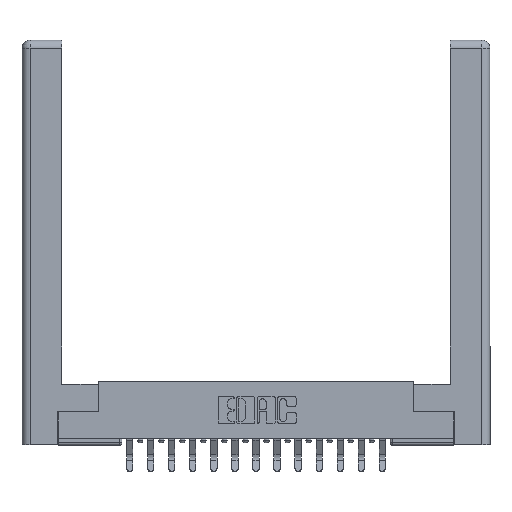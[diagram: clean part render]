
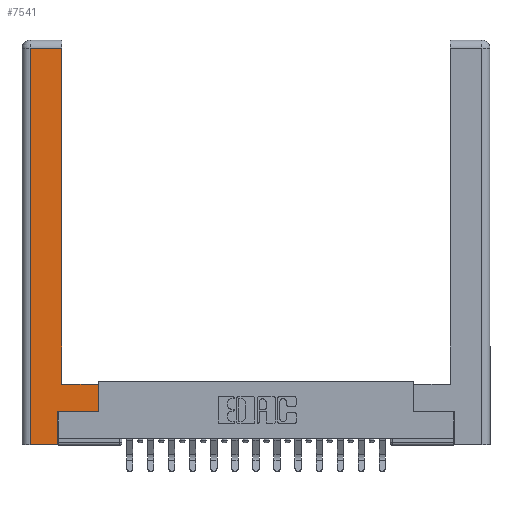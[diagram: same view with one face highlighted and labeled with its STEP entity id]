
A CAD part, top view. The second image highlights one B-rep face of the part: STEP entity #7541.
In plain terms, the highlighted planar face has unit normal (0, 0, 1).
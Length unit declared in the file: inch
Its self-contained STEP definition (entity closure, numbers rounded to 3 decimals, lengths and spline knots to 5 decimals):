
#1090 = AXIS2_PLACEMENT_3D ( 'NONE', #5129, #3698, #3776 ) ;
#1228 = CARTESIAN_POINT ( 'NONE',  ( 0.0615, 2.94, 0. ) ) ;
#1340 = VERTEX_POINT ( 'NONE', #2956 ) ;
#1878 = ORIENTED_EDGE ( 'NONE', *, *, #16406, .T. ) ;
#2419 = PLANE ( 'NONE',  #1090 ) ;
#2557 = VERTEX_POINT ( 'NONE', #12459 ) ;
#2625 = ORIENTED_EDGE ( 'NONE', *, *, #5947, .T. ) ;
#2754 = EDGE_CURVE ( 'NONE', #13485, #1340, #7481, .T. ) ;
#2850 = VECTOR ( 'NONE', #7127, 39.37008 ) ;
#2956 = CARTESIAN_POINT ( 'NONE',  ( 0.265, 0., 0. ) ) ;
#3149 = VERTEX_POINT ( 'NONE', #3576 ) ;
#3239 = ORIENTED_EDGE ( 'NONE', *, *, #15809, .T. ) ;
#3576 = CARTESIAN_POINT ( 'NONE',  ( 0.295, 0.45, 0. ) ) ;
#3641 = DIRECTION ( 'NONE',  ( 0., 1., 0. ) ) ;
#3698 = DIRECTION ( 'NONE',  ( 0., 0., -1. ) ) ;
#3776 = DIRECTION ( 'NONE',  ( -1., 0., 0. ) ) ;
#4039 = ORIENTED_EDGE ( 'NONE', *, *, #4901, .T. ) ;
#4318 = CARTESIAN_POINT ( 'NONE',  ( 0.0615, 0., 0. ) ) ;
#4670 = CARTESIAN_POINT ( 'NONE',  ( 0.565, 0.45, 0. ) ) ;
#4765 = VECTOR ( 'NONE', #6373, 39.37008 ) ;
#4901 = EDGE_CURVE ( 'NONE', #16887, #3149, #8826, .T. ) ;
#4949 = EDGE_LOOP ( 'NONE', ( #3239, #1878, #8077, #7996, #11765, #2625, #17188, #4039 ) ) ;
#5129 = CARTESIAN_POINT ( 'NONE',  ( 0., 0., 0. ) ) ;
#5903 = CARTESIAN_POINT ( 'NONE',  ( 0.0615, 2.94, 0. ) ) ;
#5947 = EDGE_CURVE ( 'NONE', #13837, #2557, #15379, .T. ) ;
#6021 = CARTESIAN_POINT ( 'NONE',  ( 0.295, 0.45, 0. ) ) ;
#6345 = LINE ( 'NONE', #17328, #15395 ) ;
#6373 = DIRECTION ( 'NONE',  ( -1., 0., 0. ) ) ;
#6860 = CARTESIAN_POINT ( 'NONE',  ( 0.565, 0.245, 0. ) ) ;
#7127 = DIRECTION ( 'NONE',  ( 0., -1., 0. ) ) ;
#7481 = LINE ( 'NONE', #15844, #9956 ) ;
#7541 = ADVANCED_FACE ( 'NONE', ( #7837 ), #2419, .F. ) ;
#7837 = FACE_OUTER_BOUND ( 'NONE', #4949, .T. ) ;
#7996 = ORIENTED_EDGE ( 'NONE', *, *, #2754, .T. ) ;
#8077 = ORIENTED_EDGE ( 'NONE', *, *, #8621, .T. ) ;
#8224 = LINE ( 'NONE', #4318, #2850 ) ;
#8266 = VECTOR ( 'NONE', #16744, 39.37008 ) ;
#8571 = DIRECTION ( 'NONE',  ( 0., 1., 0. ) ) ;
#8621 = EDGE_CURVE ( 'NONE', #16716, #13485, #8224, .T. ) ;
#8826 = LINE ( 'NONE', #6021, #4765 ) ;
#8844 = DIRECTION ( 'NONE',  ( 0., 1., 0. ) ) ;
#9018 = VERTEX_POINT ( 'NONE', #16969 ) ;
#9670 = CARTESIAN_POINT ( 'NONE',  ( 0.265, 0.245, 0. ) ) ;
#9917 = LINE ( 'NONE', #15474, #17776 ) ;
#9956 = VECTOR ( 'NONE', #14554, 39.37008 ) ;
#10528 = VECTOR ( 'NONE', #14822, 39.37008 ) ;
#11056 = CARTESIAN_POINT ( 'NONE',  ( 0.0615, 0., 0. ) ) ;
#11765 = ORIENTED_EDGE ( 'NONE', *, *, #13753, .T. ) ;
#12459 = CARTESIAN_POINT ( 'NONE',  ( 0.565, 0.245, 0. ) ) ;
#12828 = VECTOR ( 'NONE', #8844, 39.37008 ) ;
#13279 = LINE ( 'NONE', #1228, #10528 ) ;
#13485 = VERTEX_POINT ( 'NONE', #11056 ) ;
#13753 = EDGE_CURVE ( 'NONE', #1340, #13837, #6345, .T. ) ;
#13837 = VERTEX_POINT ( 'NONE', #9670 ) ;
#14554 = DIRECTION ( 'NONE',  ( 1., 0., 0. ) ) ;
#14822 = DIRECTION ( 'NONE',  ( -1., 0., 0. ) ) ;
#15379 = LINE ( 'NONE', #6860, #8266 ) ;
#15395 = VECTOR ( 'NONE', #3641, 39.37008 ) ;
#15474 = CARTESIAN_POINT ( 'NONE',  ( 0.295, 3., 0. ) ) ;
#15809 = EDGE_CURVE ( 'NONE', #3149, #9018, #9917, .T. ) ;
#15844 = CARTESIAN_POINT ( 'NONE',  ( 0.265, 0., 0. ) ) ;
#15935 = EDGE_CURVE ( 'NONE', #2557, #16887, #17107, .T. ) ;
#16067 = CARTESIAN_POINT ( 'NONE',  ( 0.565, 0.45, 0. ) ) ;
#16406 = EDGE_CURVE ( 'NONE', #9018, #16716, #13279, .T. ) ;
#16716 = VERTEX_POINT ( 'NONE', #5903 ) ;
#16744 = DIRECTION ( 'NONE',  ( 1., 0., 0. ) ) ;
#16887 = VERTEX_POINT ( 'NONE', #16067 ) ;
#16969 = CARTESIAN_POINT ( 'NONE',  ( 0.295, 2.94, 0. ) ) ;
#17107 = LINE ( 'NONE', #4670, #12828 ) ;
#17188 = ORIENTED_EDGE ( 'NONE', *, *, #15935, .T. ) ;
#17328 = CARTESIAN_POINT ( 'NONE',  ( 0.265, 0.245, 0. ) ) ;
#17776 = VECTOR ( 'NONE', #8571, 39.37008 ) ;
